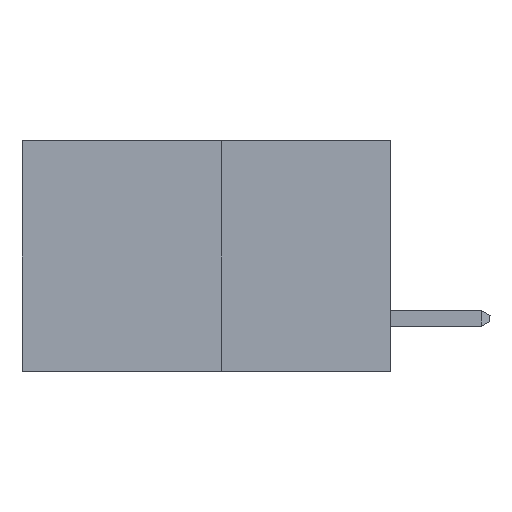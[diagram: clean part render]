
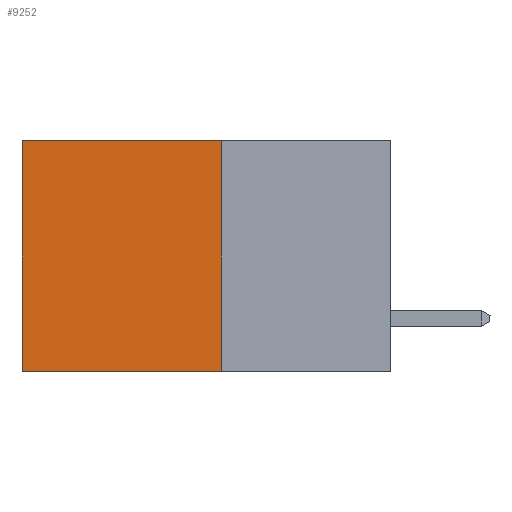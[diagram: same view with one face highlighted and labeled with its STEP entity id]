
A CAD part, left-side view. The second image highlights one B-rep face of the part: STEP entity #9252.
In plain terms, the highlighted planar face has unit normal (-1, 0, 0).
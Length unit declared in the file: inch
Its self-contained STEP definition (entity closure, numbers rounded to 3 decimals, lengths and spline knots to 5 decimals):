
#343 = CARTESIAN_POINT ( 'NONE',  ( 0.277, 0.27, 0. ) ) ;
#438 = PLANE ( 'NONE',  #5465 ) ;
#679 = EDGE_CURVE ( 'NONE', #4728, #4609, #13263, .T. ) ;
#729 = CARTESIAN_POINT ( 'NONE',  ( 0.277, 0.27, -0.37 ) ) ;
#1160 = CARTESIAN_POINT ( 'NONE',  ( 0.277, 0.27, -0.37 ) ) ;
#1425 = EDGE_CURVE ( 'NONE', #2512, #4609, #8919, .T. ) ;
#1798 = DIRECTION ( 'NONE',  ( 0., 1., 0. ) ) ;
#2183 = LINE ( 'NONE', #11782, #8586 ) ;
#2512 = VERTEX_POINT ( 'NONE', #14364 ) ;
#2597 = ORIENTED_EDGE ( 'NONE', *, *, #1425, .T. ) ;
#2617 = CARTESIAN_POINT ( 'NONE',  ( 0.277, 0.27, 0. ) ) ;
#3093 = DIRECTION ( 'NONE',  ( 0., 0., -1. ) ) ;
#3979 = ORIENTED_EDGE ( 'NONE', *, *, #679, .F. ) ;
#4247 = VECTOR ( 'NONE', #15296, 39.37008 ) ;
#4609 = VERTEX_POINT ( 'NONE', #7325 ) ;
#4728 = VERTEX_POINT ( 'NONE', #1160 ) ;
#4958 = FACE_OUTER_BOUND ( 'NONE', #10378, .T. ) ;
#5465 = AXIS2_PLACEMENT_3D ( 'NONE', #9433, #10708, #3093 ) ;
#5542 = DIRECTION ( 'NONE',  ( 0., 0., -1. ) ) ;
#5549 = VECTOR ( 'NONE', #6935, 39.37008 ) ;
#6348 = CARTESIAN_POINT ( 'NONE',  ( 0.277, 0.59, -0.37 ) ) ;
#6935 = DIRECTION ( 'NONE',  ( 0., 0., -1. ) ) ;
#7325 = CARTESIAN_POINT ( 'NONE',  ( 0.277, 0.59, -0.37 ) ) ;
#7864 = EDGE_CURVE ( 'NONE', #8695, #2512, #8071, .T. ) ;
#8071 = LINE ( 'NONE', #2617, #4247 ) ;
#8586 = VECTOR ( 'NONE', #5542, 39.37008 ) ;
#8695 = VERTEX_POINT ( 'NONE', #343 ) ;
#8919 = LINE ( 'NONE', #6348, #5549 ) ;
#9252 = ADVANCED_FACE ( 'NONE', ( #4958 ), #438, .F. ) ;
#9433 = CARTESIAN_POINT ( 'NONE',  ( 0.277, 0.27, -0.37 ) ) ;
#10378 = EDGE_LOOP ( 'NONE', ( #2597, #3979, #15794, #13110 ) ) ;
#10708 = DIRECTION ( 'NONE',  ( 1., 0., 0. ) ) ;
#11081 = VECTOR ( 'NONE', #1798, 39.37008 ) ;
#11782 = CARTESIAN_POINT ( 'NONE',  ( 0.277, 0.27, -0.37 ) ) ;
#13110 = ORIENTED_EDGE ( 'NONE', *, *, #7864, .T. ) ;
#13263 = LINE ( 'NONE', #729, #11081 ) ;
#13861 = EDGE_CURVE ( 'NONE', #8695, #4728, #2183, .T. ) ;
#14364 = CARTESIAN_POINT ( 'NONE',  ( 0.277, 0.59, 0. ) ) ;
#15296 = DIRECTION ( 'NONE',  ( 0., 1., 0. ) ) ;
#15794 = ORIENTED_EDGE ( 'NONE', *, *, #13861, .F. ) ;
